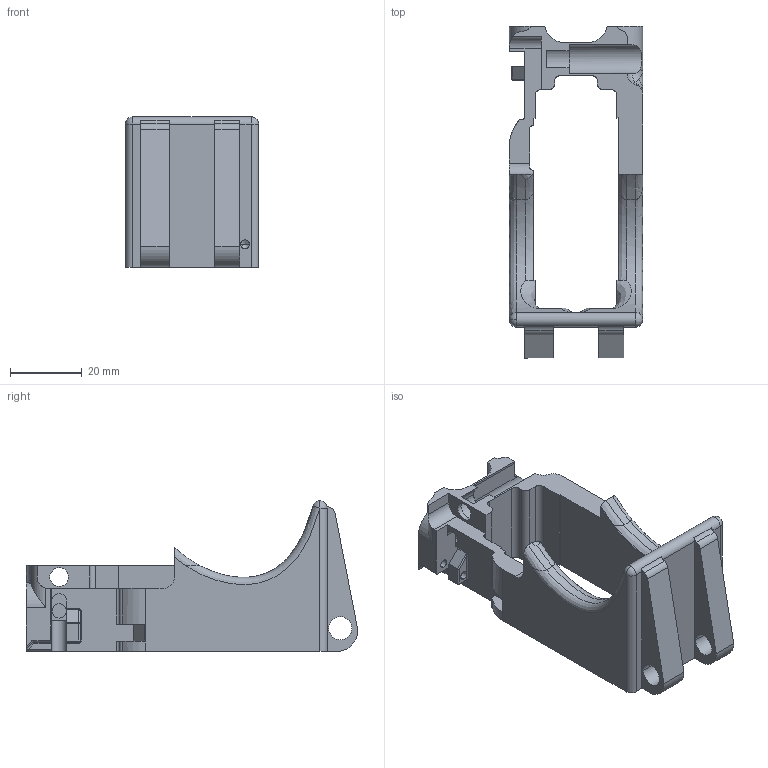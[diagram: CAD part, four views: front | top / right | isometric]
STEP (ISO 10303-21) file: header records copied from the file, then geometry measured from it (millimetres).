
FILE_DESCRIPTION (( 'STEP AP214' ), '1' );
FILE_NAME ('1Fix.STEP', '2013-09-30T13:24:24', ( 'elpi' ), ( '' ), 'SwSTEP 2.0', 'SolidWorks 2013', '' );
FILE_SCHEMA (( 'AUTOMOTIVE_DESIGN' ));
Length unit declared in the file: millimetre
Products named in the file (1): 1Fix
Bounding box: 37.13 x 92.49 x 41.85 mm (x, y, z)
Volume: 36191.8 mm3; surface area: 16440 mm2
Topology: 1 solids, 1 shells, 182 faces, 517 edges, 329 vertices
Faces by surface type: cylinder 79, plane 68, bspline 24, sphere 6, torus 3, cone 2
Entity records: 10235 total; most frequent: CARTESIAN_POINT 5624, ORIENTED_EDGE 1018, DIRECTION 894, EDGE_CURVE 509, VERTEX_POINT 329, AXIS2_PLACEMENT_3D 314, VECTOR 266, LINE 266
